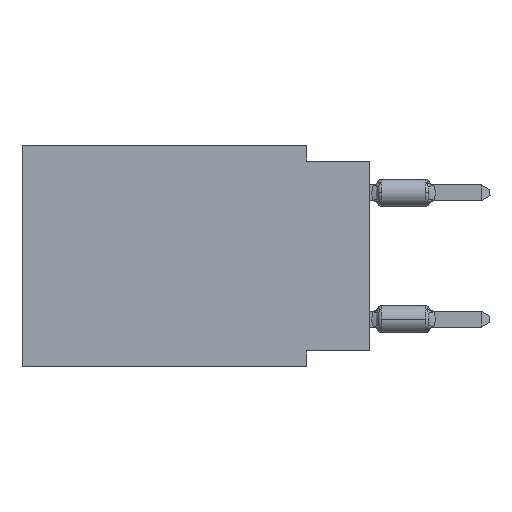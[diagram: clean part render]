
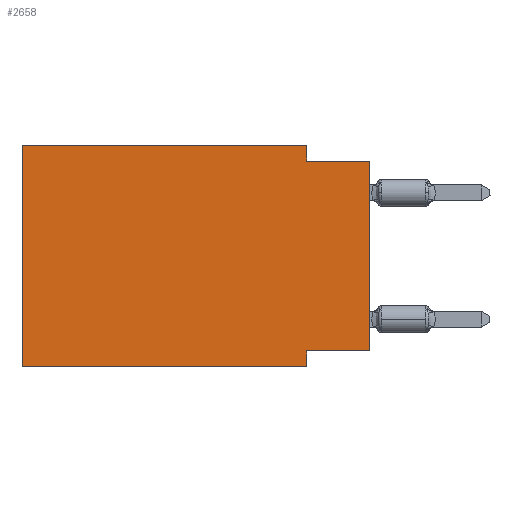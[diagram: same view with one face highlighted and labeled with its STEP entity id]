
A CAD part, left-side view. The second image highlights one B-rep face of the part: STEP entity #2658.
In plain terms, the highlighted planar face has unit normal (-1, 0, 0).
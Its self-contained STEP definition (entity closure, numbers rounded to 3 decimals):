
#72 = LINE ( 'NONE', #15231, #14519 ) ;
#82 = VERTEX_POINT ( 'NONE', #18691 ) ;
#2005 = VECTOR ( 'NONE', #3702, 1000. ) ;
#2158 = CARTESIAN_POINT ( 'NONE',  ( 0., 0., -0.635 ) ) ;
#2289 = DIRECTION ( 'NONE',  ( 0., -1., 0. ) ) ;
#2658 = ADVANCED_FACE ( 'NONE', ( #11106 ), #24079, .F. ) ;
#2669 = DIRECTION ( 'NONE',  ( 0., 1., 0. ) ) ;
#2689 = DIRECTION ( 'NONE',  ( 0., 0., 1. ) ) ;
#2809 = EDGE_CURVE ( 'NONE', #15846, #82, #17346, .T. ) ;
#3677 = VECTOR ( 'NONE', #2289, 1000. ) ;
#3702 = DIRECTION ( 'NONE',  ( 0., -1., 0. ) ) ;
#4032 = EDGE_CURVE ( 'NONE', #8599, #82, #15397, .T. ) ;
#4367 = EDGE_CURVE ( 'NONE', #16494, #10934, #72, .T. ) ;
#4547 = LINE ( 'NONE', #21733, #8842 ) ;
#4754 = CARTESIAN_POINT ( 'NONE',  ( 0., 2.54, -8.89 ) ) ;
#5599 = EDGE_LOOP ( 'NONE', ( #6166, #8991, #15077, #22964, #8797, #12757, #24522, #6514 ) ) ;
#5810 = CARTESIAN_POINT ( 'NONE',  ( 0., 0., 0. ) ) ;
#6166 = ORIENTED_EDGE ( 'NONE', *, *, #4032, .T. ) ;
#6298 = VECTOR ( 'NONE', #21287, 1000. ) ;
#6514 = ORIENTED_EDGE ( 'NONE', *, *, #11328, .F. ) ;
#6593 = EDGE_CURVE ( 'NONE', #9129, #12307, #15181, .T. ) ;
#7012 = CARTESIAN_POINT ( 'NONE',  ( 0., 13.97, 0. ) ) ;
#7888 = EDGE_CURVE ( 'NONE', #10934, #15846, #20789, .T. ) ;
#8256 = CARTESIAN_POINT ( 'NONE',  ( 0., 0., -8.255 ) ) ;
#8599 = VERTEX_POINT ( 'NONE', #16006 ) ;
#8617 = VERTEX_POINT ( 'NONE', #8649 ) ;
#8649 = CARTESIAN_POINT ( 'NONE',  ( 0., 13.97, -8.89 ) ) ;
#8797 = ORIENTED_EDGE ( 'NONE', *, *, #14645, .F. ) ;
#8842 = VECTOR ( 'NONE', #2689, 1000. ) ;
#8991 = ORIENTED_EDGE ( 'NONE', *, *, #2809, .F. ) ;
#9129 = VERTEX_POINT ( 'NONE', #16587 ) ;
#10063 = VECTOR ( 'NONE', #19019, 1000. ) ;
#10934 = VERTEX_POINT ( 'NONE', #22665 ) ;
#10976 = DIRECTION ( 'NONE',  ( 1., 0., 0. ) ) ;
#11106 = FACE_OUTER_BOUND ( 'NONE', #5599, .T. ) ;
#11194 = DIRECTION ( 'NONE',  ( 0., 0., -1. ) ) ;
#11328 = EDGE_CURVE ( 'NONE', #8599, #9129, #23465, .T. ) ;
#11568 = CARTESIAN_POINT ( 'NONE',  ( 0., 2.54, -8.89 ) ) ;
#11784 = EDGE_CURVE ( 'NONE', #8617, #12307, #15025, .T. ) ;
#12307 = VERTEX_POINT ( 'NONE', #4754 ) ;
#12757 = ORIENTED_EDGE ( 'NONE', *, *, #11784, .T. ) ;
#13502 = VECTOR ( 'NONE', #2669, 1000. ) ;
#14519 = VECTOR ( 'NONE', #17239, 1000. ) ;
#14601 = DIRECTION ( 'NONE',  ( 0., 0., -1. ) ) ;
#14645 = EDGE_CURVE ( 'NONE', #8617, #16494, #4547, .T. ) ;
#14810 = AXIS2_PLACEMENT_3D ( 'NONE', #7012, #10976, #14601 ) ;
#15025 = LINE ( 'NONE', #21590, #2005 ) ;
#15077 = ORIENTED_EDGE ( 'NONE', *, *, #7888, .F. ) ;
#15181 = LINE ( 'NONE', #11568, #22968 ) ;
#15231 = CARTESIAN_POINT ( 'NONE',  ( 0., 13.97, 0. ) ) ;
#15397 = LINE ( 'NONE', #5810, #10063 ) ;
#15846 = VERTEX_POINT ( 'NONE', #22383 ) ;
#16006 = CARTESIAN_POINT ( 'NONE',  ( 0., 0., -8.255 ) ) ;
#16494 = VERTEX_POINT ( 'NONE', #19719 ) ;
#16587 = CARTESIAN_POINT ( 'NONE',  ( 0., 2.54, -8.255 ) ) ;
#17239 = DIRECTION ( 'NONE',  ( 0., -1., 0. ) ) ;
#17346 = LINE ( 'NONE', #2158, #3677 ) ;
#18691 = CARTESIAN_POINT ( 'NONE',  ( 0., 0., -0.635 ) ) ;
#19019 = DIRECTION ( 'NONE',  ( 0., 0., 1. ) ) ;
#19719 = CARTESIAN_POINT ( 'NONE',  ( 0., 13.97, 0. ) ) ;
#20789 = LINE ( 'NONE', #21040, #6298 ) ;
#21040 = CARTESIAN_POINT ( 'NONE',  ( 0., 2.54, 0. ) ) ;
#21287 = DIRECTION ( 'NONE',  ( 0., 0., -1. ) ) ;
#21590 = CARTESIAN_POINT ( 'NONE',  ( 0., 13.97, -8.89 ) ) ;
#21733 = CARTESIAN_POINT ( 'NONE',  ( 0., 13.97, 0. ) ) ;
#22383 = CARTESIAN_POINT ( 'NONE',  ( 0., 2.54, -0.635 ) ) ;
#22665 = CARTESIAN_POINT ( 'NONE',  ( 0., 2.54, 0. ) ) ;
#22964 = ORIENTED_EDGE ( 'NONE', *, *, #4367, .F. ) ;
#22968 = VECTOR ( 'NONE', #11194, 1000. ) ;
#23465 = LINE ( 'NONE', #8256, #13502 ) ;
#24079 = PLANE ( 'NONE',  #14810 ) ;
#24522 = ORIENTED_EDGE ( 'NONE', *, *, #6593, .F. ) ;
